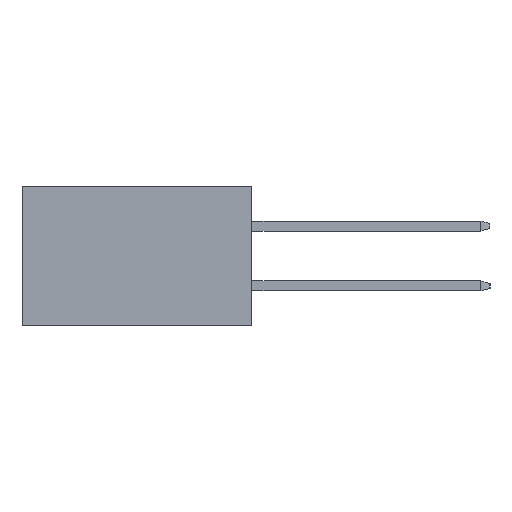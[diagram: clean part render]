
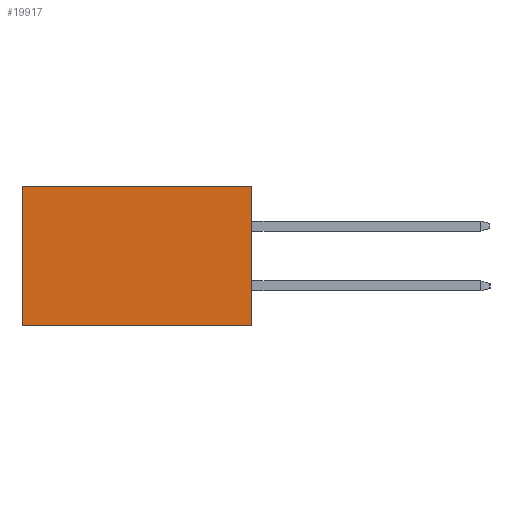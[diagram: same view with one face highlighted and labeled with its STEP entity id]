
A CAD part, left-side view. The second image highlights one B-rep face of the part: STEP entity #19917.
In plain terms, the highlighted planar face has unit normal (-1, 0, 0).
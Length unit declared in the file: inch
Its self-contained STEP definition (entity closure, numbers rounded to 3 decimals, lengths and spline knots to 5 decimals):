
#557 = ORIENTED_EDGE ( 'NONE', *, *, #19077, .F. ) ;
#763 = DIRECTION ( 'NONE',  ( 0., 0., -1. ) ) ;
#1154 = EDGE_CURVE ( 'NONE', #5732, #12345, #15017, .T. ) ;
#3086 = ORIENTED_EDGE ( 'NONE', *, *, #19442, .F. ) ;
#3980 = VECTOR ( 'NONE', #16559, 39.37008 ) ;
#4036 = CARTESIAN_POINT ( 'NONE',  ( 0.3205, 0., -0.437 ) ) ;
#4822 = VECTOR ( 'NONE', #17307, 39.37008 ) ;
#5732 = VERTEX_POINT ( 'NONE', #9097 ) ;
#6537 = CARTESIAN_POINT ( 'NONE',  ( 0.3205, 0.72, 0. ) ) ;
#7741 = LINE ( 'NONE', #4036, #18839 ) ;
#8810 = VECTOR ( 'NONE', #15120, 39.37008 ) ;
#9097 = CARTESIAN_POINT ( 'NONE',  ( 0.3205, 0., 0. ) ) ;
#9901 = PLANE ( 'NONE',  #11433 ) ;
#10210 = CARTESIAN_POINT ( 'NONE',  ( 0.3205, 0., -0.437 ) ) ;
#11176 = EDGE_CURVE ( 'NONE', #12345, #18049, #12055, .T. ) ;
#11312 = LINE ( 'NONE', #10210, #3980 ) ;
#11433 = AXIS2_PLACEMENT_3D ( 'NONE', #17015, #18867, #20730 ) ;
#12013 = FACE_OUTER_BOUND ( 'NONE', #15048, .T. ) ;
#12055 = LINE ( 'NONE', #20564, #4822 ) ;
#12345 = VERTEX_POINT ( 'NONE', #6537 ) ;
#13152 = CARTESIAN_POINT ( 'NONE',  ( 0.3205, 0., 0. ) ) ;
#13174 = ORIENTED_EDGE ( 'NONE', *, *, #1154, .T. ) ;
#15017 = LINE ( 'NONE', #13152, #8810 ) ;
#15048 = EDGE_LOOP ( 'NONE', ( #20384, #557, #3086, #13174 ) ) ;
#15120 = DIRECTION ( 'NONE',  ( 0., 1., 0. ) ) ;
#16559 = DIRECTION ( 'NONE',  ( 0., 1., 0. ) ) ;
#17015 = CARTESIAN_POINT ( 'NONE',  ( 0.3205, 0., -0.437 ) ) ;
#17307 = DIRECTION ( 'NONE',  ( 0., 0., -1. ) ) ;
#17557 = CARTESIAN_POINT ( 'NONE',  ( 0.3205, 0.72, -0.437 ) ) ;
#18049 = VERTEX_POINT ( 'NONE', #17557 ) ;
#18437 = CARTESIAN_POINT ( 'NONE',  ( 0.3205, 0., -0.437 ) ) ;
#18631 = VERTEX_POINT ( 'NONE', #18437 ) ;
#18839 = VECTOR ( 'NONE', #763, 39.37008 ) ;
#18867 = DIRECTION ( 'NONE',  ( 1., 0., 0. ) ) ;
#19077 = EDGE_CURVE ( 'NONE', #18631, #18049, #11312, .T. ) ;
#19442 = EDGE_CURVE ( 'NONE', #5732, #18631, #7741, .T. ) ;
#19917 = ADVANCED_FACE ( 'NONE', ( #12013 ), #9901, .F. ) ;
#20384 = ORIENTED_EDGE ( 'NONE', *, *, #11176, .T. ) ;
#20564 = CARTESIAN_POINT ( 'NONE',  ( 0.3205, 0.72, -0.437 ) ) ;
#20730 = DIRECTION ( 'NONE',  ( 0., 0., -1. ) ) ;
